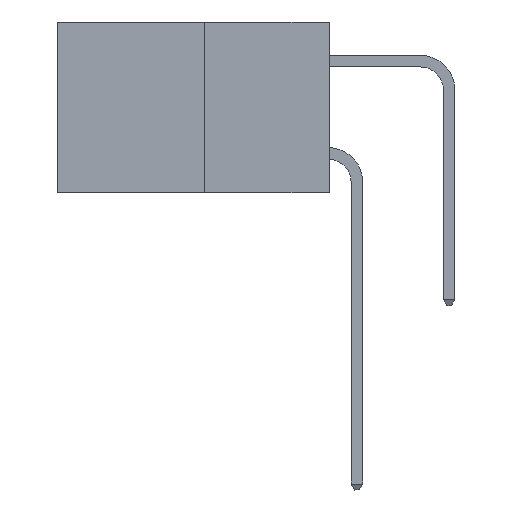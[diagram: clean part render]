
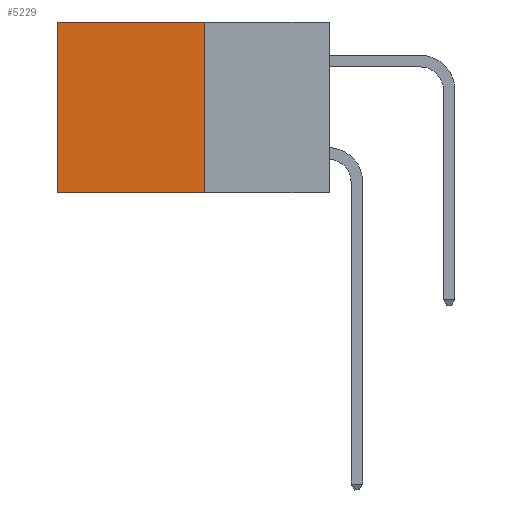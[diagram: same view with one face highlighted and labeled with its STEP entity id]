
A CAD part, left-side view. The second image highlights one B-rep face of the part: STEP entity #5229.
In plain terms, the highlighted planar face has unit normal (-1, 0, 0).
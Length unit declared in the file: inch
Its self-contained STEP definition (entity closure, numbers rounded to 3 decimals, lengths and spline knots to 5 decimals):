
#175 = CARTESIAN_POINT ( 'NONE',  ( 0.277, 0.59, -0.37 ) ) ;
#608 = VECTOR ( 'NONE', #6396, 39.37008 ) ;
#861 = DIRECTION ( 'NONE',  ( 1., 0., 0. ) ) ;
#1987 = VERTEX_POINT ( 'NONE', #6767 ) ;
#2237 = EDGE_CURVE ( 'NONE', #1987, #10710, #16613, .T. ) ;
#2238 = VERTEX_POINT ( 'NONE', #4543 ) ;
#2854 = DIRECTION ( 'NONE',  ( 0., 1., 0. ) ) ;
#3096 = CARTESIAN_POINT ( 'NONE',  ( 0.277, 0.27, -0.37 ) ) ;
#3446 = VECTOR ( 'NONE', #14575, 39.37008 ) ;
#4476 = CARTESIAN_POINT ( 'NONE',  ( 0.277, 0.27, -0.37 ) ) ;
#4543 = CARTESIAN_POINT ( 'NONE',  ( 0.277, 0.59, 0. ) ) ;
#4935 = EDGE_CURVE ( 'NONE', #2238, #11111, #7780, .T. ) ;
#5229 = ADVANCED_FACE ( 'NONE', ( #14939 ), #19952, .F. ) ;
#6396 = DIRECTION ( 'NONE',  ( 0., 0., -1. ) ) ;
#6701 = VECTOR ( 'NONE', #9611, 39.37008 ) ;
#6767 = CARTESIAN_POINT ( 'NONE',  ( 0.277, 0.27, 0. ) ) ;
#7780 = LINE ( 'NONE', #175, #3446 ) ;
#7947 = CARTESIAN_POINT ( 'NONE',  ( 0.277, 0.59, -0.37 ) ) ;
#8542 = LINE ( 'NONE', #18810, #16934 ) ;
#9611 = DIRECTION ( 'NONE',  ( 0., 1., 0. ) ) ;
#10335 = ORIENTED_EDGE ( 'NONE', *, *, #4935, .T. ) ;
#10692 = ORIENTED_EDGE ( 'NONE', *, *, #18210, .F. ) ;
#10710 = VERTEX_POINT ( 'NONE', #11709 ) ;
#11111 = VERTEX_POINT ( 'NONE', #7947 ) ;
#11598 = ORIENTED_EDGE ( 'NONE', *, *, #2237, .F. ) ;
#11709 = CARTESIAN_POINT ( 'NONE',  ( 0.277, 0.27, -0.37 ) ) ;
#12110 = DIRECTION ( 'NONE',  ( 0., 0., -1. ) ) ;
#13306 = ORIENTED_EDGE ( 'NONE', *, *, #17470, .T. ) ;
#14543 = EDGE_LOOP ( 'NONE', ( #10335, #10692, #11598, #13306 ) ) ;
#14575 = DIRECTION ( 'NONE',  ( 0., 0., -1. ) ) ;
#14939 = FACE_OUTER_BOUND ( 'NONE', #14543, .T. ) ;
#14978 = AXIS2_PLACEMENT_3D ( 'NONE', #16793, #861, #12110 ) ;
#15173 = LINE ( 'NONE', #3096, #6701 ) ;
#16613 = LINE ( 'NONE', #4476, #608 ) ;
#16793 = CARTESIAN_POINT ( 'NONE',  ( 0.277, 0.27, -0.37 ) ) ;
#16934 = VECTOR ( 'NONE', #2854, 39.37008 ) ;
#17470 = EDGE_CURVE ( 'NONE', #1987, #2238, #8542, .T. ) ;
#18210 = EDGE_CURVE ( 'NONE', #10710, #11111, #15173, .T. ) ;
#18810 = CARTESIAN_POINT ( 'NONE',  ( 0.277, 0.27, 0. ) ) ;
#19952 = PLANE ( 'NONE',  #14978 ) ;
